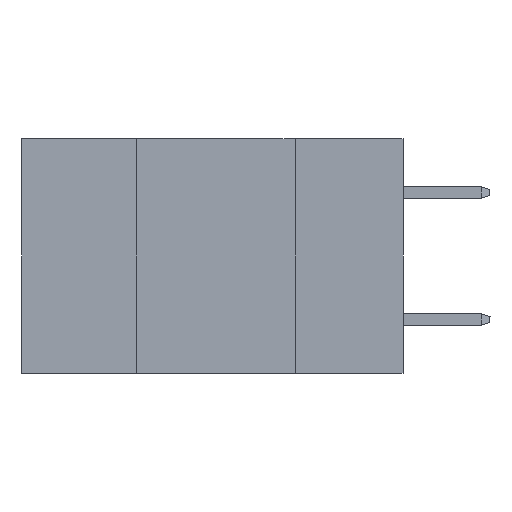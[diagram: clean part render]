
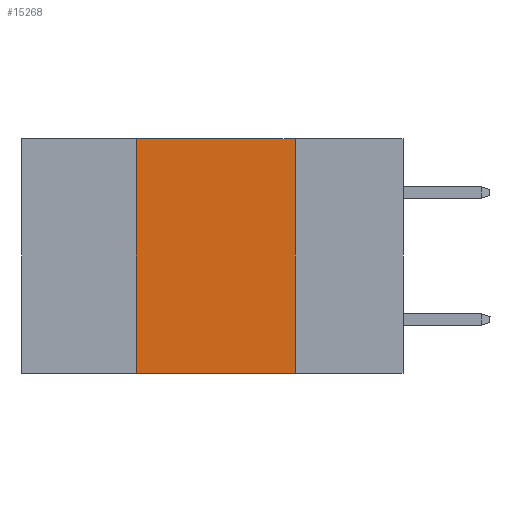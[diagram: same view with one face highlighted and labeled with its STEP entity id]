
A CAD part, left-side view. The second image highlights one B-rep face of the part: STEP entity #15268.
In plain terms, the highlighted planar face has unit normal (-1, 0, 0).
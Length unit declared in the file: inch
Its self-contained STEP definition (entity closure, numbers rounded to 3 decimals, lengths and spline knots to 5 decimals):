
#247 = LINE ( 'NONE', #24363, #9016 ) ;
#476 = CARTESIAN_POINT ( 'NONE',  ( 0., 0.17, 0. ) ) ;
#1156 = CARTESIAN_POINT ( 'NONE',  ( 0., 0.17, 0. ) ) ;
#2665 = VERTEX_POINT ( 'NONE', #13549 ) ;
#2857 = FACE_OUTER_BOUND ( 'NONE', #24741, .T. ) ;
#4272 = LINE ( 'NONE', #6254, #25307 ) ;
#5525 = EDGE_CURVE ( 'NONE', #20885, #2665, #25140, .T. ) ;
#6254 = CARTESIAN_POINT ( 'NONE',  ( 0., 0.42, 0. ) ) ;
#6312 = DIRECTION ( 'NONE',  ( 0., -1., 0. ) ) ;
#6627 = DIRECTION ( 'NONE',  ( 0., -1., 0. ) ) ;
#6762 = LINE ( 'NONE', #18354, #15765 ) ;
#7088 = DIRECTION ( 'NONE',  ( 0., 0., -1. ) ) ;
#8158 = EDGE_CURVE ( 'NONE', #23219, #23998, #4272, .T. ) ;
#9016 = VECTOR ( 'NONE', #6312, 39.37008 ) ;
#11069 = ORIENTED_EDGE ( 'NONE', *, *, #13625, .T. ) ;
#11529 = EDGE_CURVE ( 'NONE', #23998, #20885, #247, .T. ) ;
#11774 = ORIENTED_EDGE ( 'NONE', *, *, #5525, .F. ) ;
#13549 = CARTESIAN_POINT ( 'NONE',  ( 0., 0.17, -0.37 ) ) ;
#13625 = EDGE_CURVE ( 'NONE', #23219, #2665, #6762, .T. ) ;
#14311 = DIRECTION ( 'NONE',  ( 0., 0., 1. ) ) ;
#15268 = ADVANCED_FACE ( 'NONE', ( #2857 ), #21067, .F. ) ;
#15765 = VECTOR ( 'NONE', #6627, 39.37008 ) ;
#17498 = ORIENTED_EDGE ( 'NONE', *, *, #8158, .F. ) ;
#17903 = AXIS2_PLACEMENT_3D ( 'NONE', #23168, #19471, #19336 ) ;
#18354 = CARTESIAN_POINT ( 'NONE',  ( 0., 0.6, -0.37 ) ) ;
#19336 = DIRECTION ( 'NONE',  ( 0., 0., -1. ) ) ;
#19471 = DIRECTION ( 'NONE',  ( 1., 0., 0. ) ) ;
#19640 = ORIENTED_EDGE ( 'NONE', *, *, #11529, .F. ) ;
#19999 = VECTOR ( 'NONE', #7088, 39.37008 ) ;
#20044 = CARTESIAN_POINT ( 'NONE',  ( 0., 0.42, 0. ) ) ;
#20885 = VERTEX_POINT ( 'NONE', #476 ) ;
#21067 = PLANE ( 'NONE',  #17903 ) ;
#22793 = CARTESIAN_POINT ( 'NONE',  ( 0., 0.42, -0.37 ) ) ;
#23168 = CARTESIAN_POINT ( 'NONE',  ( 0., 0.6, 0. ) ) ;
#23219 = VERTEX_POINT ( 'NONE', #22793 ) ;
#23998 = VERTEX_POINT ( 'NONE', #20044 ) ;
#24363 = CARTESIAN_POINT ( 'NONE',  ( 0., 0.6, 0. ) ) ;
#24741 = EDGE_LOOP ( 'NONE', ( #11774, #19640, #17498, #11069 ) ) ;
#25140 = LINE ( 'NONE', #1156, #19999 ) ;
#25307 = VECTOR ( 'NONE', #14311, 39.37008 ) ;
